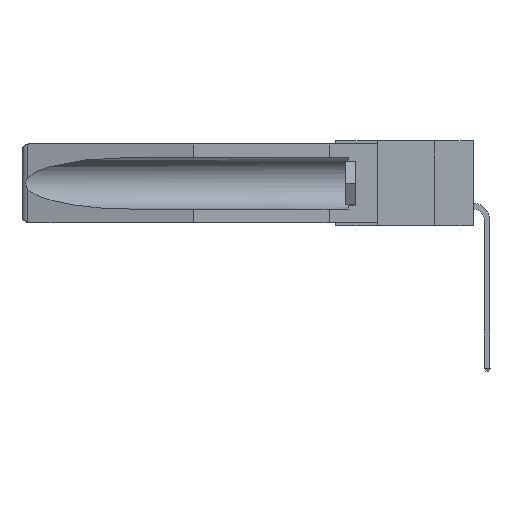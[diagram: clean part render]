
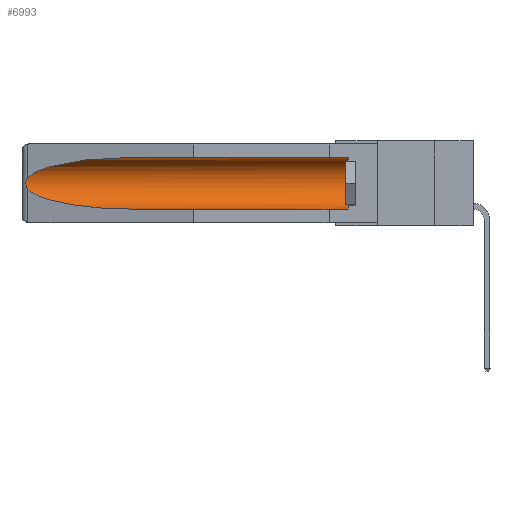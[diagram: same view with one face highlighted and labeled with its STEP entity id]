
A CAD part, left-side view. The second image highlights one B-rep face of the part: STEP entity #6993.
In plain terms, the highlighted cylindrical face has radius 2.857 mm (diameter 5.715 mm), a partial arc.
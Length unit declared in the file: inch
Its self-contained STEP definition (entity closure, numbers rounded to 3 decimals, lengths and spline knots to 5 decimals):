
#173 = EDGE_CURVE ( 'NONE', #1323, #21519, #3998, .T. ) ;
#234 = CARTESIAN_POINT ( 'NONE',  ( 0.26537, 1.52718, -0.19328 ) ) ;
#432 = CARTESIAN_POINT ( 'NONE',  ( 0.26654, 1.53092, -0.15636 ) ) ;
#753 = CARTESIAN_POINT ( 'NONE',  ( 0.155, 1.07973, -0.059 ) ) ;
#1323 = VERTEX_POINT ( 'NONE', #7529 ) ;
#2387 = VECTOR ( 'NONE', #6892, 39.37008 ) ;
#3409 = VERTEX_POINT ( 'NONE', #19973 ) ;
#3561 = LINE ( 'NONE', #14224, #15212 ) ;
#3998 =( BOUNDED_CURVE ( )  B_SPLINE_CURVE ( 3, ( #25383, #11440, #20760, #20457 ),
 .UNSPECIFIED., .F., .F. ) 
 B_SPLINE_CURVE_WITH_KNOTS ( ( 4, 4 ),
 ( 0.1948, 1.5708 ),
 .UNSPECIFIED. ) 
 CURVE ( )  GEOMETRIC_REPRESENTATION_ITEM ( )  RATIONAL_B_SPLINE_CURVE ( ( 1., 0.848, 0.848, 1. ) ) 
 REPRESENTATION_ITEM ( '' )  );
#4099 = ORIENTED_EDGE ( 'NONE', *, *, #13827, .T. ) ;
#4187 = AXIS2_PLACEMENT_3D ( 'NONE', #17016, #26386, #5739 ) ;
#4671 = EDGE_LOOP ( 'NONE', ( #21475, #4912, #13422, #13597, #5440, #4099 ) ) ;
#4815 = CIRCLE ( 'NONE', #4187, 0.1125 ) ;
#4912 = ORIENTED_EDGE ( 'NONE', *, *, #21873, .T. ) ;
#5058 = CARTESIAN_POINT ( 'NONE',  ( 0.2675, 1.53308, -0.16763 ) ) ;
#5440 = ORIENTED_EDGE ( 'NONE', *, *, #10987, .T. ) ;
#5458 = CARTESIAN_POINT ( 'NONE',  ( 0.21114, 1.30732, -0.059 ) ) ;
#5739 = DIRECTION ( 'NONE',  ( 0., 0., 1. ) ) ;
#5825 = CARTESIAN_POINT ( 'NONE',  ( 0.26537, 1.52718, -0.14972 ) ) ;
#5967 = DIRECTION ( 'NONE',  ( 0., 0., 1. ) ) ;
#6069 = CARTESIAN_POINT ( 'NONE',  ( 0.155, -0.30754, -0.1715 ) ) ;
#6892 = DIRECTION ( 'NONE',  ( 0., 1., 0. ) ) ;
#6993 = ADVANCED_FACE ( 'NONE', ( #10878 ), #16338, .F. ) ;
#7453 = CARTESIAN_POINT ( 'NONE',  ( 0.2675, 1.53308, -0.17534 ) ) ;
#7529 = CARTESIAN_POINT ( 'NONE',  ( 0.26537, 1.52718, -0.19328 ) ) ;
#8573 = LINE ( 'NONE', #21095, #2387 ) ;
#9705 = CARTESIAN_POINT ( 'NONE',  ( 0.26655, 1.53094, -0.18657 ) ) ;
#10312 = CARTESIAN_POINT ( 'NONE',  ( 0.26537, 1.52718, -0.14972 ) ) ;
#10878 = FACE_OUTER_BOUND ( 'NONE', #4671, .T. ) ;
#10987 = EDGE_CURVE ( 'NONE', #11968, #17159, #4815, .T. ) ;
#11440 = CARTESIAN_POINT ( 'NONE',  ( 0.25451, 1.48313, -0.24835 ) ) ;
#11968 = VERTEX_POINT ( 'NONE', #16312 ) ;
#12136 = AXIS2_PLACEMENT_3D ( 'NONE', #6069, #15310, #5967 ) ;
#13422 = ORIENTED_EDGE ( 'NONE', *, *, #173, .T. ) ;
#13597 = ORIENTED_EDGE ( 'NONE', *, *, #22165, .F. ) ;
#13827 = EDGE_CURVE ( 'NONE', #17159, #3409, #8573, .T. ) ;
#14171 = EDGE_CURVE ( 'NONE', #3409, #23746, #18498, .T. ) ;
#14224 = CARTESIAN_POINT ( 'NONE',  ( 0.155, -0.30754, -0.284 ) ) ;
#14289 = CARTESIAN_POINT ( 'NONE',  ( 0.2673, 1.5327, -0.16383 ) ) ;
#15013 = CARTESIAN_POINT ( 'NONE',  ( 0.25451, 1.48313, -0.09465 ) ) ;
#15212 = VECTOR ( 'NONE', #18974, 39.37008 ) ;
#15310 = DIRECTION ( 'NONE',  ( 0., 1., 0. ) ) ;
#16312 = CARTESIAN_POINT ( 'NONE',  ( 0.155, 0.126, -0.284 ) ) ;
#16338 = CYLINDRICAL_SURFACE ( 'NONE', #12136, 0.1125 ) ;
#16520 = CARTESIAN_POINT ( 'NONE',  ( 0.26597, 1.52961, -0.15275 ) ) ;
#17016 = CARTESIAN_POINT ( 'NONE',  ( 0.155, 0.126, -0.1715 ) ) ;
#17159 = VERTEX_POINT ( 'NONE', #26784 ) ;
#18498 =( BOUNDED_CURVE ( )  B_SPLINE_CURVE ( 3, ( #753, #5458, #15013, #10312 ),
 .UNSPECIFIED., .F., .F. ) 
 B_SPLINE_CURVE_WITH_KNOTS ( ( 4, 4 ),
 ( 4.71239, 6.08839 ),
 .UNSPECIFIED. ) 
 CURVE ( )  GEOMETRIC_REPRESENTATION_ITEM ( )  RATIONAL_B_SPLINE_CURVE ( ( 1., 0.848, 0.848, 1. ) ) 
 REPRESENTATION_ITEM ( '' )  );
#18974 = DIRECTION ( 'NONE',  ( 0., 1., 0. ) ) ;
#19973 = CARTESIAN_POINT ( 'NONE',  ( 0.155, 1.07973, -0.059 ) ) ;
#20457 = CARTESIAN_POINT ( 'NONE',  ( 0.155, 1.07973, -0.284 ) ) ;
#20760 = CARTESIAN_POINT ( 'NONE',  ( 0.21114, 1.30732, -0.284 ) ) ;
#21074 = CARTESIAN_POINT ( 'NONE',  ( 0.26597, 1.5296, -0.19026 ) ) ;
#21095 = CARTESIAN_POINT ( 'NONE',  ( 0.155, -0.30754, -0.059 ) ) ;
#21383 = CARTESIAN_POINT ( 'NONE',  ( 0.2673, 1.53269, -0.17917 ) ) ;
#21475 = ORIENTED_EDGE ( 'NONE', *, *, #14171, .T. ) ;
#21519 = VERTEX_POINT ( 'NONE', #29734 ) ;
#21671 = B_SPLINE_CURVE_WITH_KNOTS ( 'NONE', 3,
 ( #28255, #16520, #432, #14289, #5058, #7453, #21383, #9705, #21074, #234 ),
 .UNSPECIFIED., .F., .F.,
 ( 4, 2, 2, 2, 4 ),
 ( 0., 0.00029, 0.00058, 0.00087, 0.00117 ),
 .UNSPECIFIED. ) ;
#21873 = EDGE_CURVE ( 'NONE', #23746, #1323, #21671, .T. ) ;
#22165 = EDGE_CURVE ( 'NONE', #11968, #21519, #3561, .T. ) ;
#23746 = VERTEX_POINT ( 'NONE', #5825 ) ;
#25383 = CARTESIAN_POINT ( 'NONE',  ( 0.26537, 1.52718, -0.19328 ) ) ;
#26386 = DIRECTION ( 'NONE',  ( 0., -1., 0. ) ) ;
#26784 = CARTESIAN_POINT ( 'NONE',  ( 0.155, 0.126, -0.059 ) ) ;
#28255 = CARTESIAN_POINT ( 'NONE',  ( 0.26537, 1.52718, -0.14972 ) ) ;
#29734 = CARTESIAN_POINT ( 'NONE',  ( 0.155, 1.07973, -0.284 ) ) ;
